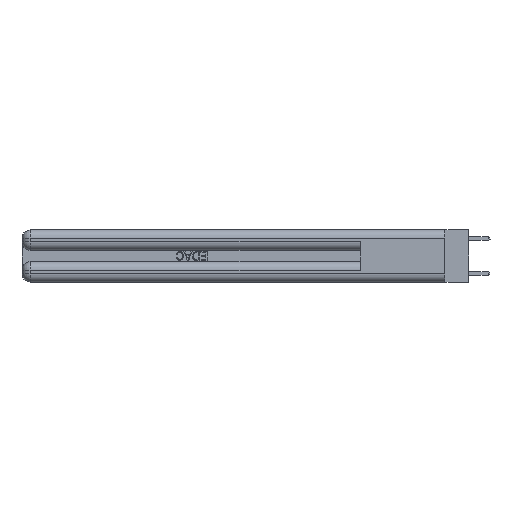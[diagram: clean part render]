
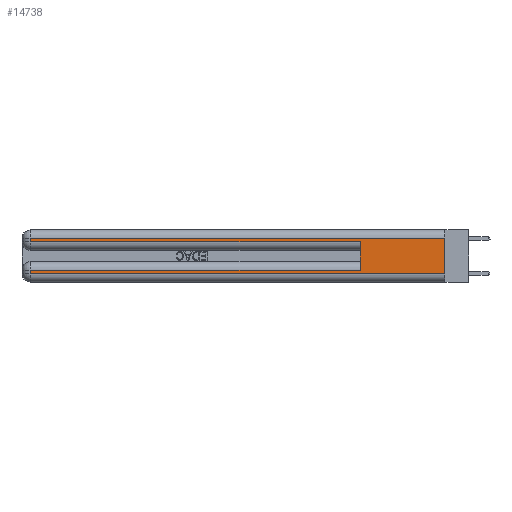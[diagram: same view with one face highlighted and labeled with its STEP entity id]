
A CAD part, left-side view. The second image highlights one B-rep face of the part: STEP entity #14738.
In plain terms, the highlighted planar face has unit normal (-1, 0, 0).
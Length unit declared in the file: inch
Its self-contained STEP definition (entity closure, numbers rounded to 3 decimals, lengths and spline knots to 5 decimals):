
#505 = EDGE_CURVE ( 'NONE', #32173, #6433, #23357, .T. ) ;
#1527 = EDGE_CURVE ( 'NONE', #8043, #14230, #30389, .T. ) ;
#1583 = DIRECTION ( 'NONE',  ( 0., 1., 0. ) ) ;
#2137 = DIRECTION ( 'NONE',  ( 1., 0., 0. ) ) ;
#2741 = CARTESIAN_POINT ( 'NONE',  ( 0., 2.94, 0.31 ) ) ;
#3894 = ORIENTED_EDGE ( 'NONE', *, *, #1527, .T. ) ;
#4309 = EDGE_LOOP ( 'NONE', ( #8737, #35199, #25691, #29345, #13522, #31758, #15414, #3894 ) ) ;
#5642 = EDGE_CURVE ( 'NONE', #35261, #8043, #22221, .T. ) ;
#6052 = CARTESIAN_POINT ( 'NONE',  ( 0., 0., 0.37 ) ) ;
#6336 = CARTESIAN_POINT ( 'NONE',  ( 0., 0.6, 0.145 ) ) ;
#6433 = VERTEX_POINT ( 'NONE', #18898 ) ;
#8043 = VERTEX_POINT ( 'NONE', #8539 ) ;
#8228 = DIRECTION ( 'NONE',  ( 0., -1., 0. ) ) ;
#8298 = VECTOR ( 'NONE', #29451, 39.37008 ) ;
#8539 = CARTESIAN_POINT ( 'NONE',  ( 0., 2.94, 0.06 ) ) ;
#8737 = ORIENTED_EDGE ( 'NONE', *, *, #19497, .F. ) ;
#9568 = VECTOR ( 'NONE', #20465, 39.37008 ) ;
#10014 = VECTOR ( 'NONE', #19862, 39.37008 ) ;
#10477 = CARTESIAN_POINT ( 'NONE',  ( 0., 0., 0.37 ) ) ;
#10893 = LINE ( 'NONE', #6052, #10014 ) ;
#11408 = LINE ( 'NONE', #6336, #32115 ) ;
#12119 = CARTESIAN_POINT ( 'NONE',  ( 0., 0., 0.31 ) ) ;
#12734 = VECTOR ( 'NONE', #18248, 39.37008 ) ;
#12912 = VECTOR ( 'NONE', #1583, 39.37008 ) ;
#13522 = ORIENTED_EDGE ( 'NONE', *, *, #28866, .F. ) ;
#13711 = VERTEX_POINT ( 'NONE', #12119 ) ;
#14230 = VERTEX_POINT ( 'NONE', #22373 ) ;
#14738 = ADVANCED_FACE ( 'NONE', ( #22527 ), #21398, .F. ) ;
#15414 = ORIENTED_EDGE ( 'NONE', *, *, #5642, .T. ) ;
#15482 = CARTESIAN_POINT ( 'NONE',  ( 0., 2.94, 0.37 ) ) ;
#15767 = VERTEX_POINT ( 'NONE', #30927 ) ;
#16543 = LINE ( 'NONE', #18544, #8298 ) ;
#18220 = CARTESIAN_POINT ( 'NONE',  ( 0., 2.94, 0.37 ) ) ;
#18248 = DIRECTION ( 'NONE',  ( 0., 0., -1. ) ) ;
#18544 = CARTESIAN_POINT ( 'NONE',  ( 0., 0., 0.31 ) ) ;
#18898 = CARTESIAN_POINT ( 'NONE',  ( 0., 0.6, 0.285 ) ) ;
#19497 = EDGE_CURVE ( 'NONE', #13711, #14230, #10893, .T. ) ;
#19862 = DIRECTION ( 'NONE',  ( 0., 0., -1. ) ) ;
#20465 = DIRECTION ( 'NONE',  ( 0., -1., 0. ) ) ;
#21398 = PLANE ( 'NONE',  #25036 ) ;
#21509 = DIRECTION ( 'NONE',  ( 0., 0., -1. ) ) ;
#21865 = VERTEX_POINT ( 'NONE', #2741 ) ;
#22221 = LINE ( 'NONE', #18220, #28478 ) ;
#22236 = EDGE_CURVE ( 'NONE', #15767, #35261, #33579, .T. ) ;
#22373 = CARTESIAN_POINT ( 'NONE',  ( 0., 0., 0.06 ) ) ;
#22527 = FACE_OUTER_BOUND ( 'NONE', #4309, .T. ) ;
#22945 = DIRECTION ( 'NONE',  ( 0., 0., 1. ) ) ;
#23357 = LINE ( 'NONE', #27319, #24202 ) ;
#23694 = CARTESIAN_POINT ( 'NONE',  ( 0., 0., 0.085 ) ) ;
#24202 = VECTOR ( 'NONE', #8228, 39.37008 ) ;
#25036 = AXIS2_PLACEMENT_3D ( 'NONE', #10477, #2137, #21509 ) ;
#25691 = ORIENTED_EDGE ( 'NONE', *, *, #28111, .T. ) ;
#27319 = CARTESIAN_POINT ( 'NONE',  ( 0., 0., 0.285 ) ) ;
#28111 = EDGE_CURVE ( 'NONE', #21865, #32173, #34225, .T. ) ;
#28478 = VECTOR ( 'NONE', #31817, 39.37008 ) ;
#28866 = EDGE_CURVE ( 'NONE', #15767, #6433, #11408, .T. ) ;
#29187 = EDGE_CURVE ( 'NONE', #13711, #21865, #16543, .T. ) ;
#29345 = ORIENTED_EDGE ( 'NONE', *, *, #505, .T. ) ;
#29451 = DIRECTION ( 'NONE',  ( 0., 1., 0. ) ) ;
#30040 = CARTESIAN_POINT ( 'NONE',  ( 0., 2.94, 0.285 ) ) ;
#30389 = LINE ( 'NONE', #33767, #9568 ) ;
#30927 = CARTESIAN_POINT ( 'NONE',  ( 0., 0.6, 0.085 ) ) ;
#31758 = ORIENTED_EDGE ( 'NONE', *, *, #22236, .T. ) ;
#31817 = DIRECTION ( 'NONE',  ( 0., 0., -1. ) ) ;
#32058 = CARTESIAN_POINT ( 'NONE',  ( 0., 2.94, 0.085 ) ) ;
#32115 = VECTOR ( 'NONE', #22945, 39.37008 ) ;
#32173 = VERTEX_POINT ( 'NONE', #30040 ) ;
#33579 = LINE ( 'NONE', #23694, #12912 ) ;
#33767 = CARTESIAN_POINT ( 'NONE',  ( 0., 0., 0.06 ) ) ;
#34225 = LINE ( 'NONE', #15482, #12734 ) ;
#35199 = ORIENTED_EDGE ( 'NONE', *, *, #29187, .T. ) ;
#35261 = VERTEX_POINT ( 'NONE', #32058 ) ;
